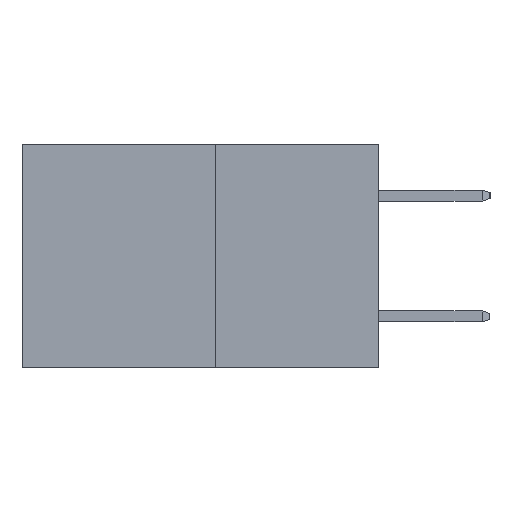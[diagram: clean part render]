
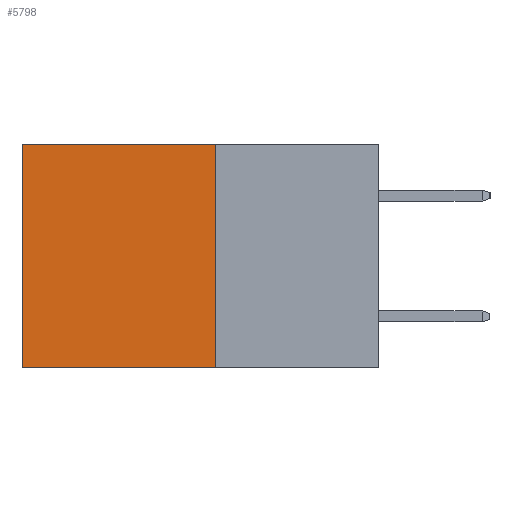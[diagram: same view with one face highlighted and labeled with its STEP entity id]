
A CAD part, left-side view. The second image highlights one B-rep face of the part: STEP entity #5798.
In plain terms, the highlighted planar face has unit normal (-1, 0, 0).
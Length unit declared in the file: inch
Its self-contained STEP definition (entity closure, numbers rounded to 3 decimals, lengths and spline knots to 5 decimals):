
#513 = LINE ( 'NONE', #12122, #7136 ) ;
#571 = VERTEX_POINT ( 'NONE', #11075 ) ;
#986 = EDGE_CURVE ( 'NONE', #15697, #7192, #7130, .T. ) ;
#1114 = CARTESIAN_POINT ( 'NONE',  ( 0.277, 0.27, -0.37 ) ) ;
#3020 = EDGE_CURVE ( 'NONE', #571, #13166, #3951, .T. ) ;
#3951 = LINE ( 'NONE', #8590, #13222 ) ;
#4421 = ORIENTED_EDGE ( 'NONE', *, *, #986, .T. ) ;
#4509 = VECTOR ( 'NONE', #5313, 39.37008 ) ;
#4582 = ORIENTED_EDGE ( 'NONE', *, *, #12313, .F. ) ;
#5313 = DIRECTION ( 'NONE',  ( 0., 1., 0. ) ) ;
#5339 = CARTESIAN_POINT ( 'NONE',  ( 0.277, 0.59, -0.37 ) ) ;
#5655 = ORIENTED_EDGE ( 'NONE', *, *, #3020, .F. ) ;
#5798 = ADVANCED_FACE ( 'NONE', ( #8157 ), #7227, .F. ) ;
#6432 = ORIENTED_EDGE ( 'NONE', *, *, #13904, .T. ) ;
#7010 = EDGE_LOOP ( 'NONE', ( #4421, #4582, #5655, #6432 ) ) ;
#7130 = LINE ( 'NONE', #16402, #11065 ) ;
#7136 = VECTOR ( 'NONE', #13403, 39.37008 ) ;
#7191 = DIRECTION ( 'NONE',  ( 0., 0., -1. ) ) ;
#7192 = VERTEX_POINT ( 'NONE', #5339 ) ;
#7224 = DIRECTION ( 'NONE',  ( 1., 0., 0. ) ) ;
#7227 = PLANE ( 'NONE',  #9359 ) ;
#7303 = CARTESIAN_POINT ( 'NONE',  ( 0.277, 0.27, -0.37 ) ) ;
#8157 = FACE_OUTER_BOUND ( 'NONE', #7010, .T. ) ;
#8491 = DIRECTION ( 'NONE',  ( 0., 0., -1. ) ) ;
#8590 = CARTESIAN_POINT ( 'NONE',  ( 0.277, 0.27, -0.37 ) ) ;
#9359 = AXIS2_PLACEMENT_3D ( 'NONE', #7303, #7224, #7191 ) ;
#10501 = CARTESIAN_POINT ( 'NONE',  ( 0.277, 0.59, 0. ) ) ;
#11065 = VECTOR ( 'NONE', #11658, 39.37008 ) ;
#11075 = CARTESIAN_POINT ( 'NONE',  ( 0.277, 0.27, 0. ) ) ;
#11560 = LINE ( 'NONE', #13942, #4509 ) ;
#11658 = DIRECTION ( 'NONE',  ( 0., 0., -1. ) ) ;
#12122 = CARTESIAN_POINT ( 'NONE',  ( 0.277, 0.27, 0. ) ) ;
#12313 = EDGE_CURVE ( 'NONE', #13166, #7192, #11560, .T. ) ;
#13166 = VERTEX_POINT ( 'NONE', #1114 ) ;
#13222 = VECTOR ( 'NONE', #8491, 39.37008 ) ;
#13403 = DIRECTION ( 'NONE',  ( 0., 1., 0. ) ) ;
#13904 = EDGE_CURVE ( 'NONE', #571, #15697, #513, .T. ) ;
#13942 = CARTESIAN_POINT ( 'NONE',  ( 0.277, 0.27, -0.37 ) ) ;
#15697 = VERTEX_POINT ( 'NONE', #10501 ) ;
#16402 = CARTESIAN_POINT ( 'NONE',  ( 0.277, 0.59, -0.37 ) ) ;
